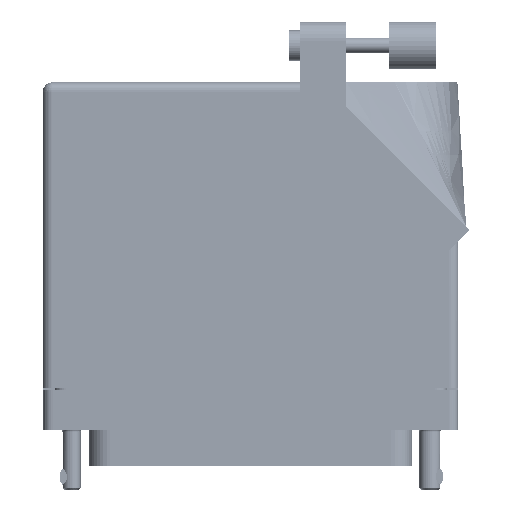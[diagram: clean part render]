
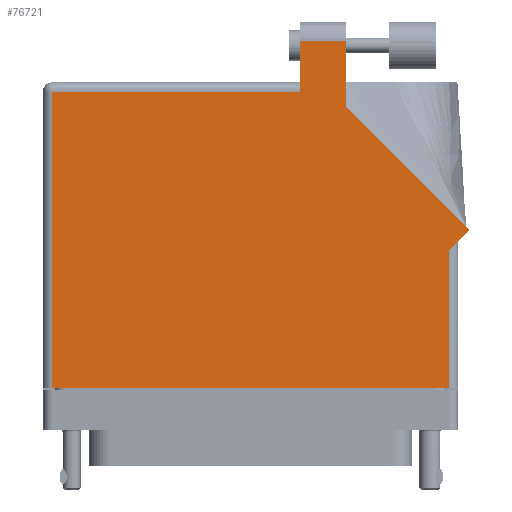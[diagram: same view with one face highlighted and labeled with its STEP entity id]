
A CAD part, front view. The second image highlights one B-rep face of the part: STEP entity #76721.
In plain terms, the highlighted face is planar.
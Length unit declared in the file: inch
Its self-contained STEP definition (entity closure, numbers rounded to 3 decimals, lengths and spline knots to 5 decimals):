
#7 = LINE ( 'NONE', #95360, #17969 ) ;
#265 = LINE ( 'NONE', #8611, #50956 ) ;
#343 = VECTOR ( 'NONE', #64419, 39.37008 ) ;
#2759 = CARTESIAN_POINT ( 'NONE',  ( -1.3155, -0.1, 0.765 ) ) ;
#4278 = DIRECTION ( 'NONE',  ( 0., -1., 0. ) ) ;
#7195 = ORIENTED_EDGE ( 'NONE', *, *, #64989, .T. ) ;
#7556 = DIRECTION ( 'NONE',  ( -1., 0., 0. ) ) ;
#8054 = CARTESIAN_POINT ( 'NONE',  ( 1.44821, 0.95071, 0.765 ) ) ;
#8611 = CARTESIAN_POINT ( 'NONE',  ( 0.3275, 2.205, 0.765 ) ) ;
#11254 = LINE ( 'NONE', #97236, #55219 ) ;
#13723 = VERTEX_POINT ( 'NONE', #50425 ) ;
#14339 = DIRECTION ( 'NONE',  ( -0.707, 0.707, 0. ) ) ;
#16230 = CARTESIAN_POINT ( 'NONE',  ( -1.3155, 1.868, 0.765 ) ) ;
#16378 = LINE ( 'NONE', #22656, #25454 ) ;
#16733 = EDGE_CURVE ( 'NONE', #95768, #76270, #72117, .T. ) ;
#17494 = ORIENTED_EDGE ( 'NONE', *, *, #100515, .T. ) ;
#17719 = AXIS2_PLACEMENT_3D ( 'NONE', #59790, #95027, #52994 ) ;
#17969 = VECTOR ( 'NONE', #23989, 39.37008 ) ;
#22656 = CARTESIAN_POINT ( 'NONE',  ( 1.3775, 0.88, 0.765 ) ) ;
#23148 = VECTOR ( 'NONE', #62083, 39.37008 ) ;
#23153 = FACE_OUTER_BOUND ( 'NONE', #29758, .T. ) ;
#23989 = DIRECTION ( 'NONE',  ( -1., 0., 0. ) ) ;
#25454 = VECTOR ( 'NONE', #79928, 39.37008 ) ;
#26345 = ORIENTED_EDGE ( 'NONE', *, *, #58505, .T. ) ;
#29134 = ORIENTED_EDGE ( 'NONE', *, *, #46713, .T. ) ;
#29758 = EDGE_LOOP ( 'NONE', ( #85614, #90998, #66261, #7195, #26345, #73923, #29134, #17494, #58670 ) ) ;
#30662 = EDGE_CURVE ( 'NONE', #85413, #56036, #67751, .T. ) ;
#33154 = LINE ( 'NONE', #98269, #343 ) ;
#35248 = EDGE_CURVE ( 'NONE', #66206, #85413, #265, .T. ) ;
#39022 = CARTESIAN_POINT ( 'NONE',  ( 0.3275, 1.93, 0.765 ) ) ;
#41868 = CARTESIAN_POINT ( 'NONE',  ( 1.44821, 0.95071, 0.765 ) ) ;
#45596 = CARTESIAN_POINT ( 'NONE',  ( 0.3275, 1.868, 0.765 ) ) ;
#46695 = VERTEX_POINT ( 'NONE', #16230 ) ;
#46713 = EDGE_CURVE ( 'NONE', #13723, #96377, #64144, .T. ) ;
#48144 = CARTESIAN_POINT ( 'NONE',  ( 0.6345, 2.205, 0.765 ) ) ;
#50425 = CARTESIAN_POINT ( 'NONE',  ( 1.3155, -0.1, 0.765 ) ) ;
#50956 = VECTOR ( 'NONE', #7556, 39.37008 ) ;
#52085 = CARTESIAN_POINT ( 'NONE',  ( 0.6345, 1.76442, 0.765 ) ) ;
#52994 = DIRECTION ( 'NONE',  ( -1., 0., 0. ) ) ;
#54141 = DIRECTION ( 'NONE',  ( 0., -1., 0. ) ) ;
#55219 = VECTOR ( 'NONE', #56595, 39.37008 ) ;
#56036 = VERTEX_POINT ( 'NONE', #45596 ) ;
#56595 = DIRECTION ( 'NONE',  ( 1., 0., 0. ) ) ;
#58505 = EDGE_CURVE ( 'NONE', #46695, #64074, #90263, .T. ) ;
#58670 = ORIENTED_EDGE ( 'NONE', *, *, #16733, .T. ) ;
#59790 = CARTESIAN_POINT ( 'NONE',  ( -1.3775, 1.93, 0.765 ) ) ;
#62083 = DIRECTION ( 'NONE',  ( 0., 1., 0. ) ) ;
#64074 = VERTEX_POINT ( 'NONE', #96387 ) ;
#64144 = LINE ( 'NONE', #94894, #23148 ) ;
#64419 = DIRECTION ( 'NONE',  ( 0., 1., 0. ) ) ;
#64989 = EDGE_CURVE ( 'NONE', #56036, #46695, #7, .T. ) ;
#66206 = VERTEX_POINT ( 'NONE', #48144 ) ;
#66261 = ORIENTED_EDGE ( 'NONE', *, *, #30662, .T. ) ;
#67186 = VECTOR ( 'NONE', #54141, 39.37008 ) ;
#67751 = LINE ( 'NONE', #39022, #67186 ) ;
#72117 = LINE ( 'NONE', #8054, #90789 ) ;
#73650 = CARTESIAN_POINT ( 'NONE',  ( 0.3275, 2.205, 0.765 ) ) ;
#73923 = ORIENTED_EDGE ( 'NONE', *, *, #84957, .T. ) ;
#76270 = VERTEX_POINT ( 'NONE', #52085 ) ;
#76721 = ADVANCED_FACE ( 'NONE', ( #23153 ), #102849, .F. ) ;
#79928 = DIRECTION ( 'NONE',  ( 0.707, 0.707, 0. ) ) ;
#84957 = EDGE_CURVE ( 'NONE', #64074, #13723, #11254, .T. ) ;
#85143 = EDGE_CURVE ( 'NONE', #76270, #66206, #33154, .T. ) ;
#85413 = VERTEX_POINT ( 'NONE', #73650 ) ;
#85614 = ORIENTED_EDGE ( 'NONE', *, *, #85143, .T. ) ;
#90263 = LINE ( 'NONE', #2759, #90295 ) ;
#90295 = VECTOR ( 'NONE', #4278, 39.37008 ) ;
#90789 = VECTOR ( 'NONE', #14339, 39.37008 ) ;
#90998 = ORIENTED_EDGE ( 'NONE', *, *, #35248, .T. ) ;
#93616 = CARTESIAN_POINT ( 'NONE',  ( 1.3155, 0.818, 0.765 ) ) ;
#94894 = CARTESIAN_POINT ( 'NONE',  ( 1.3155, 0.88, 0.765 ) ) ;
#95027 = DIRECTION ( 'NONE',  ( 0., 0., -1. ) ) ;
#95360 = CARTESIAN_POINT ( 'NONE',  ( -1.3775, 1.868, 0.765 ) ) ;
#95768 = VERTEX_POINT ( 'NONE', #41868 ) ;
#96377 = VERTEX_POINT ( 'NONE', #93616 ) ;
#96387 = CARTESIAN_POINT ( 'NONE',  ( -1.3155, -0.1, 0.765 ) ) ;
#97236 = CARTESIAN_POINT ( 'NONE',  ( -1.3775, -0.1, 0.765 ) ) ;
#98269 = CARTESIAN_POINT ( 'NONE',  ( 0.6345, 1.76442, 0.765 ) ) ;
#100515 = EDGE_CURVE ( 'NONE', #96377, #95768, #16378, .T. ) ;
#102849 = PLANE ( 'NONE',  #17719 ) ;
